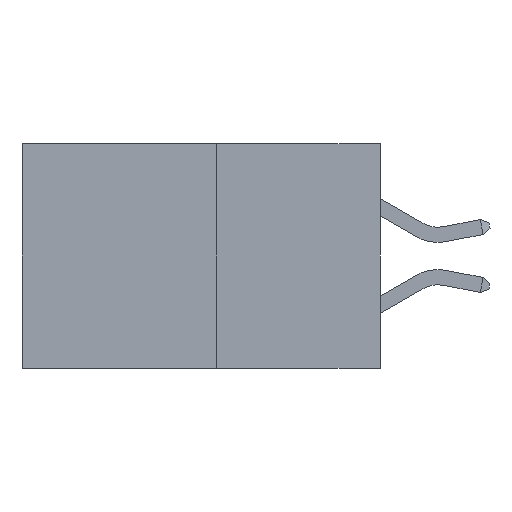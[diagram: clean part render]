
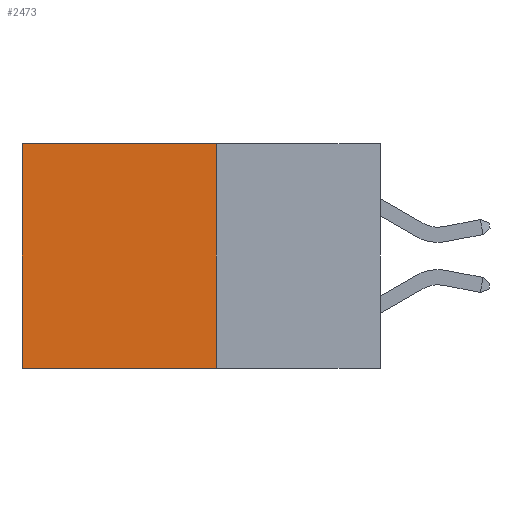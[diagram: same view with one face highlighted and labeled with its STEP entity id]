
A CAD part, left-side view. The second image highlights one B-rep face of the part: STEP entity #2473.
In plain terms, the highlighted planar face has unit normal (-1, 0, 0).
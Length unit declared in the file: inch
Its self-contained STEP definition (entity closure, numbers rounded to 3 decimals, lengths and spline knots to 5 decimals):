
#230 = VECTOR ( 'NONE', #1699, 39.37008 ) ;
#304 = ORIENTED_EDGE ( 'NONE', *, *, #7895, .F. ) ;
#522 = VERTEX_POINT ( 'NONE', #7383 ) ;
#1142 = DIRECTION ( 'NONE',  ( 0., 0., -1. ) ) ;
#1187 = EDGE_CURVE ( 'NONE', #8202, #6653, #9113, .T. ) ;
#1699 = DIRECTION ( 'NONE',  ( 0., 1., 0. ) ) ;
#2144 = CARTESIAN_POINT ( 'NONE',  ( 0.277, 0.27, 0. ) ) ;
#2468 = CARTESIAN_POINT ( 'NONE',  ( 0.277, 0.27, -0.37 ) ) ;
#2473 = ADVANCED_FACE ( 'NONE', ( #7517 ), #6865, .F. ) ;
#2588 = EDGE_CURVE ( 'NONE', #5139, #6653, #4840, .T. ) ;
#2658 = DIRECTION ( 'NONE',  ( 0., 0., -1. ) ) ;
#2728 = VECTOR ( 'NONE', #2658, 39.37008 ) ;
#2988 = VECTOR ( 'NONE', #8099, 39.37008 ) ;
#3100 = EDGE_CURVE ( 'NONE', #522, #5139, #4177, .T. ) ;
#3468 = VECTOR ( 'NONE', #5688, 39.37008 ) ;
#3930 = EDGE_LOOP ( 'NONE', ( #6531, #4038, #304, #5254 ) ) ;
#4038 = ORIENTED_EDGE ( 'NONE', *, *, #1187, .F. ) ;
#4177 = LINE ( 'NONE', #2144, #230 ) ;
#4804 = LINE ( 'NONE', #5423, #2728 ) ;
#4840 = LINE ( 'NONE', #8299, #2988 ) ;
#5139 = VERTEX_POINT ( 'NONE', #8325 ) ;
#5254 = ORIENTED_EDGE ( 'NONE', *, *, #3100, .T. ) ;
#5423 = CARTESIAN_POINT ( 'NONE',  ( 0.277, 0.27, -0.37 ) ) ;
#5441 = CARTESIAN_POINT ( 'NONE',  ( 0.277, 0.27, -0.37 ) ) ;
#5688 = DIRECTION ( 'NONE',  ( 0., 1., 0. ) ) ;
#6215 = CARTESIAN_POINT ( 'NONE',  ( 0.277, 0.59, -0.37 ) ) ;
#6531 = ORIENTED_EDGE ( 'NONE', *, *, #2588, .T. ) ;
#6653 = VERTEX_POINT ( 'NONE', #6215 ) ;
#6855 = DIRECTION ( 'NONE',  ( 1., 0., 0. ) ) ;
#6865 = PLANE ( 'NONE',  #8414 ) ;
#7383 = CARTESIAN_POINT ( 'NONE',  ( 0.277, 0.27, 0. ) ) ;
#7517 = FACE_OUTER_BOUND ( 'NONE', #3930, .T. ) ;
#7799 = CARTESIAN_POINT ( 'NONE',  ( 0.277, 0.27, -0.37 ) ) ;
#7895 = EDGE_CURVE ( 'NONE', #522, #8202, #4804, .T. ) ;
#8099 = DIRECTION ( 'NONE',  ( 0., 0., -1. ) ) ;
#8202 = VERTEX_POINT ( 'NONE', #7799 ) ;
#8299 = CARTESIAN_POINT ( 'NONE',  ( 0.277, 0.59, -0.37 ) ) ;
#8325 = CARTESIAN_POINT ( 'NONE',  ( 0.277, 0.59, 0. ) ) ;
#8414 = AXIS2_PLACEMENT_3D ( 'NONE', #5441, #6855, #1142 ) ;
#9113 = LINE ( 'NONE', #2468, #3468 ) ;
